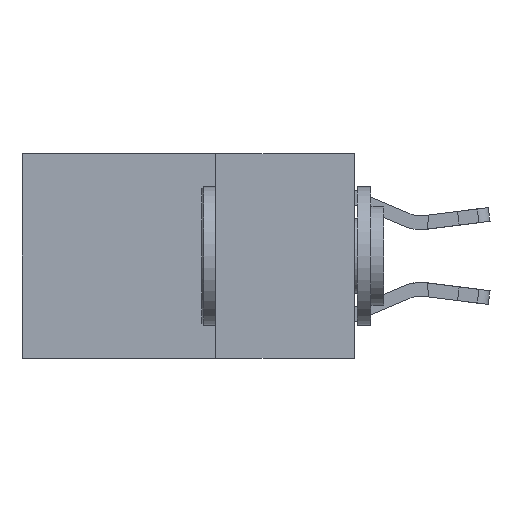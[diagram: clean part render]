
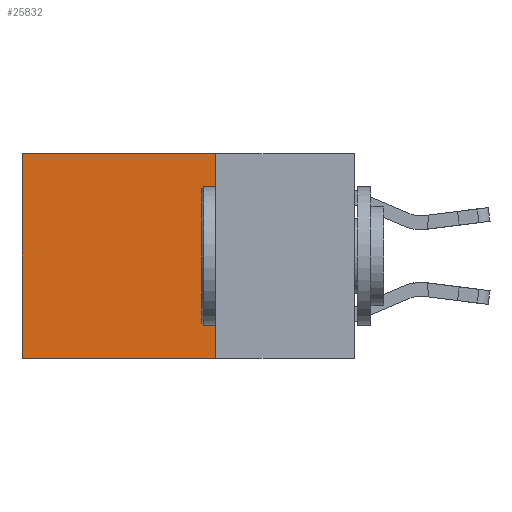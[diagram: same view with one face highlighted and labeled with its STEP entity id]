
A CAD part, left-side view. The second image highlights one B-rep face of the part: STEP entity #25832.
In plain terms, the highlighted planar face has unit normal (-1, 0, 0).
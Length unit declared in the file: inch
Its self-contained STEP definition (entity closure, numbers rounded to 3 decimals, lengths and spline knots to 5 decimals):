
#263 = CARTESIAN_POINT ( 'NONE',  ( 0.2625, 0.6, 0. ) ) ;
#795 = DIRECTION ( 'NONE',  ( 0., 0., -1. ) ) ;
#1274 = VERTEX_POINT ( 'NONE', #5463 ) ;
#2038 = DIRECTION ( 'NONE',  ( 0., 1., 0. ) ) ;
#2081 = CARTESIAN_POINT ( 'NONE',  ( 0.2625, 0.25, -0.37 ) ) ;
#2247 = ORIENTED_EDGE ( 'NONE', *, *, #24552, .F. ) ;
#2858 = CARTESIAN_POINT ( 'NONE',  ( 0.2625, 0.6, 0. ) ) ;
#2863 = VECTOR ( 'NONE', #2038, 39.37008 ) ;
#3472 = DIRECTION ( 'NONE',  ( 1., 0., 0. ) ) ;
#4250 = EDGE_CURVE ( 'NONE', #1274, #11123, #6914, .T. ) ;
#4687 = CARTESIAN_POINT ( 'NONE',  ( 0.2625, 0.25, 0. ) ) ;
#4699 = EDGE_CURVE ( 'NONE', #23490, #29343, #6880, .T. ) ;
#5463 = CARTESIAN_POINT ( 'NONE',  ( 0.2625, 0.25, 0. ) ) ;
#5544 = FACE_OUTER_BOUND ( 'NONE', #18701, .T. ) ;
#6119 = ORIENTED_EDGE ( 'NONE', *, *, #4250, .F. ) ;
#6880 = LINE ( 'NONE', #2858, #24839 ) ;
#6914 = LINE ( 'NONE', #4687, #17221 ) ;
#9713 = CARTESIAN_POINT ( 'NONE',  ( 0.2625, 0.25, 0. ) ) ;
#10001 = CARTESIAN_POINT ( 'NONE',  ( 0.2625, 0.25, -0.37 ) ) ;
#10805 = LINE ( 'NONE', #10953, #2863 ) ;
#10953 = CARTESIAN_POINT ( 'NONE',  ( 0.2625, 0.25, 0. ) ) ;
#11123 = VERTEX_POINT ( 'NONE', #10001 ) ;
#11538 = DIRECTION ( 'NONE',  ( 0., 0., -1. ) ) ;
#12145 = ORIENTED_EDGE ( 'NONE', *, *, #4699, .T. ) ;
#14026 = DIRECTION ( 'NONE',  ( 0., 0., -1. ) ) ;
#14625 = PLANE ( 'NONE',  #15920 ) ;
#15613 = DIRECTION ( 'NONE',  ( 0., 1., 0. ) ) ;
#15920 = AXIS2_PLACEMENT_3D ( 'NONE', #9713, #3472, #795 ) ;
#17221 = VECTOR ( 'NONE', #11538, 39.37008 ) ;
#18701 = EDGE_LOOP ( 'NONE', ( #12145, #2247, #6119, #23924 ) ) ;
#18752 = EDGE_CURVE ( 'NONE', #1274, #23490, #10805, .T. ) ;
#21923 = CARTESIAN_POINT ( 'NONE',  ( 0.2625, 0.6, -0.37 ) ) ;
#23490 = VERTEX_POINT ( 'NONE', #263 ) ;
#23924 = ORIENTED_EDGE ( 'NONE', *, *, #18752, .T. ) ;
#24377 = LINE ( 'NONE', #2081, #24877 ) ;
#24552 = EDGE_CURVE ( 'NONE', #11123, #29343, #24377, .T. ) ;
#24839 = VECTOR ( 'NONE', #14026, 39.37008 ) ;
#24877 = VECTOR ( 'NONE', #15613, 39.37008 ) ;
#25832 = ADVANCED_FACE ( 'NONE', ( #5544 ), #14625, .F. ) ;
#29343 = VERTEX_POINT ( 'NONE', #21923 ) ;
